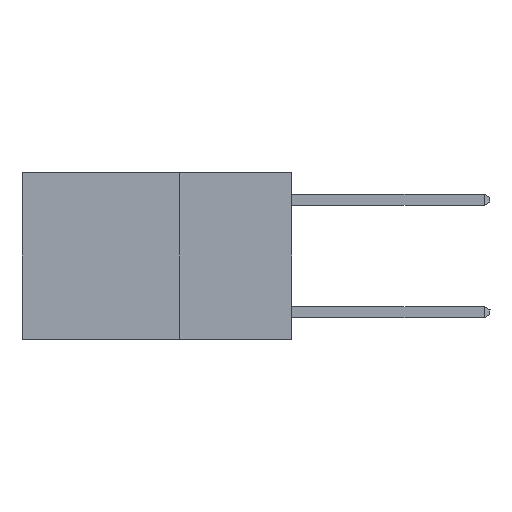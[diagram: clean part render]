
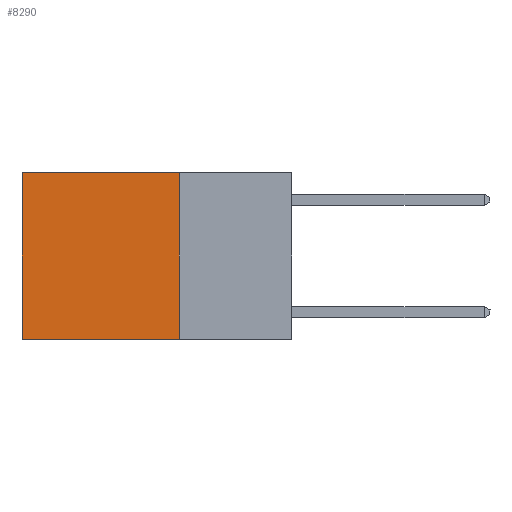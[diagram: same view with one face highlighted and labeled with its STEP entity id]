
A CAD part, left-side view. The second image highlights one B-rep face of the part: STEP entity #8290.
In plain terms, the highlighted planar face has unit normal (-1, 0, 0).
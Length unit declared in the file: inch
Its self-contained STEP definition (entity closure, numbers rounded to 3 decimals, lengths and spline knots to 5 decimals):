
#183 = AXIS2_PLACEMENT_3D ( 'NONE', #3110, #10263, #4208 ) ;
#400 = EDGE_CURVE ( 'NONE', #2173, #8518, #5404, .T. ) ;
#730 = VECTOR ( 'NONE', #8063, 39.37008 ) ;
#812 = CARTESIAN_POINT ( 'NONE',  ( 0.2625, 0.25, 0. ) ) ;
#892 = CARTESIAN_POINT ( 'NONE',  ( 0.2625, 0.25, 0. ) ) ;
#1004 = LINE ( 'NONE', #892, #11476 ) ;
#1740 = ORIENTED_EDGE ( 'NONE', *, *, #7014, .F. ) ;
#2173 = VERTEX_POINT ( 'NONE', #7726 ) ;
#2275 = DIRECTION ( 'NONE',  ( 0., 1., 0. ) ) ;
#2319 = CARTESIAN_POINT ( 'NONE',  ( 0.2625, 0.25, -0.37 ) ) ;
#3110 = CARTESIAN_POINT ( 'NONE',  ( 0.2625, 0.25, 0. ) ) ;
#4060 = DIRECTION ( 'NONE',  ( 0., 0., -1. ) ) ;
#4174 = LINE ( 'NONE', #12206, #11524 ) ;
#4208 = DIRECTION ( 'NONE',  ( 0., 0., -1. ) ) ;
#4226 = DIRECTION ( 'NONE',  ( 0., 0., -1. ) ) ;
#5373 = EDGE_LOOP ( 'NONE', ( #12422, #10349, #1740, #12764 ) ) ;
#5404 = LINE ( 'NONE', #2319, #12672 ) ;
#7014 = EDGE_CURVE ( 'NONE', #10582, #2173, #1004, .T. ) ;
#7469 = FACE_OUTER_BOUND ( 'NONE', #5373, .T. ) ;
#7726 = CARTESIAN_POINT ( 'NONE',  ( 0.2625, 0.25, -0.37 ) ) ;
#8063 = DIRECTION ( 'NONE',  ( 0., 1., 0. ) ) ;
#8276 = PLANE ( 'NONE',  #183 ) ;
#8290 = ADVANCED_FACE ( 'NONE', ( #7469 ), #8276, .F. ) ;
#8493 = VERTEX_POINT ( 'NONE', #11493 ) ;
#8518 = VERTEX_POINT ( 'NONE', #11544 ) ;
#9288 = CARTESIAN_POINT ( 'NONE',  ( 0.2625, 0.25, 0. ) ) ;
#10263 = DIRECTION ( 'NONE',  ( 1., 0., 0. ) ) ;
#10349 = ORIENTED_EDGE ( 'NONE', *, *, #400, .F. ) ;
#10432 = EDGE_CURVE ( 'NONE', #10582, #8493, #11413, .T. ) ;
#10582 = VERTEX_POINT ( 'NONE', #9288 ) ;
#11413 = LINE ( 'NONE', #812, #730 ) ;
#11476 = VECTOR ( 'NONE', #4060, 39.37008 ) ;
#11493 = CARTESIAN_POINT ( 'NONE',  ( 0.2625, 0.6, 0. ) ) ;
#11524 = VECTOR ( 'NONE', #4226, 39.37008 ) ;
#11544 = CARTESIAN_POINT ( 'NONE',  ( 0.2625, 0.6, -0.37 ) ) ;
#11899 = EDGE_CURVE ( 'NONE', #8493, #8518, #4174, .T. ) ;
#12206 = CARTESIAN_POINT ( 'NONE',  ( 0.2625, 0.6, 0. ) ) ;
#12422 = ORIENTED_EDGE ( 'NONE', *, *, #11899, .T. ) ;
#12672 = VECTOR ( 'NONE', #2275, 39.37008 ) ;
#12764 = ORIENTED_EDGE ( 'NONE', *, *, #10432, .T. ) ;
